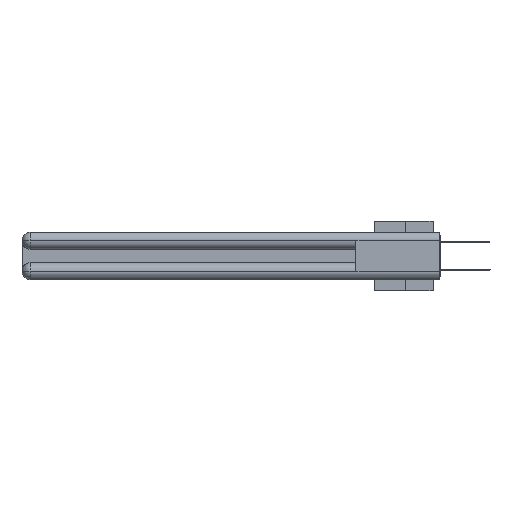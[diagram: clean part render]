
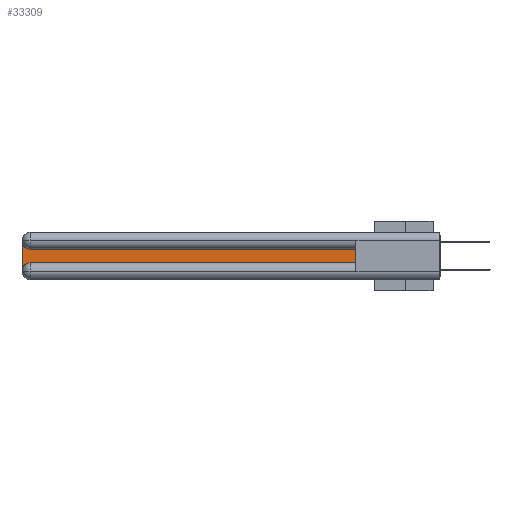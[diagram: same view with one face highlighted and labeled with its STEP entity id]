
A CAD part, left-side view. The second image highlights one B-rep face of the part: STEP entity #33309.
In plain terms, the highlighted planar face has unit normal (-1, 0, 0).
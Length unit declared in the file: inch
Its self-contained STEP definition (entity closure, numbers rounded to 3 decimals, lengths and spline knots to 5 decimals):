
#169 = DIRECTION ( 'NONE',  ( 0., 1., 0. ) ) ;
#691 = CARTESIAN_POINT ( 'NONE',  ( 0.075, 0.6, -0.2175 ) ) ;
#1352 = VECTOR ( 'NONE', #169, 39.37008 ) ;
#3128 = EDGE_CURVE ( 'NONE', #10000, #4557, #29777, .T. ) ;
#3247 = CARTESIAN_POINT ( 'NONE',  ( 0.075, 0.6, -0.2175 ) ) ;
#3289 = CARTESIAN_POINT ( 'NONE',  ( 0.075, 3., -0.1225 ) ) ;
#3720 = DIRECTION ( 'NONE',  ( 1., 0., 0. ) ) ;
#4289 = CARTESIAN_POINT ( 'NONE',  ( 0.075, 3., -0.2775 ) ) ;
#4380 = ORIENTED_EDGE ( 'NONE', *, *, #30515, .T. ) ;
#4533 = LINE ( 'NONE', #16848, #8865 ) ;
#4557 = VERTEX_POINT ( 'NONE', #12154 ) ;
#5357 = ORIENTED_EDGE ( 'NONE', *, *, #26463, .T. ) ;
#5626 = EDGE_CURVE ( 'NONE', #35240, #22213, #4533, .T. ) ;
#5837 = CIRCLE ( 'NONE', #23917, 0.06 ) ;
#6052 = VERTEX_POINT ( 'NONE', #20536 ) ;
#6240 = LINE ( 'NONE', #11932, #23591 ) ;
#6322 = DIRECTION ( 'NONE',  ( 0., 0., -1. ) ) ;
#6680 = VECTOR ( 'NONE', #30129, 39.37008 ) ;
#8865 = VECTOR ( 'NONE', #13929, 39.37008 ) ;
#9356 = ORIENTED_EDGE ( 'NONE', *, *, #15688, .T. ) ;
#10000 = VERTEX_POINT ( 'NONE', #25457 ) ;
#10992 = CARTESIAN_POINT ( 'NONE',  ( 0.075, 0.6, -0.1225 ) ) ;
#11683 = LINE ( 'NONE', #3247, #6680 ) ;
#11932 = CARTESIAN_POINT ( 'NONE',  ( 0.075, 3., -0.2175 ) ) ;
#12154 = CARTESIAN_POINT ( 'NONE',  ( 0.075, 2.94, -0.1225 ) ) ;
#13929 = DIRECTION ( 'NONE',  ( 0., -1., 0. ) ) ;
#14477 = AXIS2_PLACEMENT_3D ( 'NONE', #3289, #33278, #21062 ) ;
#15664 = ORIENTED_EDGE ( 'NONE', *, *, #3128, .T. ) ;
#15688 = EDGE_CURVE ( 'NONE', #6052, #34232, #6240, .T. ) ;
#16848 = CARTESIAN_POINT ( 'NONE',  ( 0.075, 0.6, -0.2175 ) ) ;
#18567 = EDGE_LOOP ( 'NONE', ( #15664, #28429, #9356, #4380, #30590, #5357 ) ) ;
#20536 = CARTESIAN_POINT ( 'NONE',  ( 0.075, 3., -0.0625 ) ) ;
#21062 = DIRECTION ( 'NONE',  ( 0., 0., -1. ) ) ;
#21448 = PLANE ( 'NONE',  #14477 ) ;
#21680 = CARTESIAN_POINT ( 'NONE',  ( 0.075, 2.94, -0.0625 ) ) ;
#22213 = VERTEX_POINT ( 'NONE', #691 ) ;
#23053 = AXIS2_PLACEMENT_3D ( 'NONE', #24832, #24655, #6322 ) ;
#23591 = VECTOR ( 'NONE', #23807, 39.37008 ) ;
#23807 = DIRECTION ( 'NONE',  ( 0., 0., -1. ) ) ;
#23823 = DIRECTION ( 'NONE',  ( 0., 0., -1. ) ) ;
#23917 = AXIS2_PLACEMENT_3D ( 'NONE', #21680, #3720, #23823 ) ;
#24146 = EDGE_CURVE ( 'NONE', #4557, #6052, #5837, .T. ) ;
#24655 = DIRECTION ( 'NONE',  ( 1., 0., 0. ) ) ;
#24832 = CARTESIAN_POINT ( 'NONE',  ( 0.075, 2.94, -0.2775 ) ) ;
#25457 = CARTESIAN_POINT ( 'NONE',  ( 0.075, 0.6, -0.1225 ) ) ;
#25613 = CARTESIAN_POINT ( 'NONE',  ( 0.075, 2.94, -0.2175 ) ) ;
#26463 = EDGE_CURVE ( 'NONE', #22213, #10000, #11683, .T. ) ;
#28429 = ORIENTED_EDGE ( 'NONE', *, *, #24146, .T. ) ;
#29777 = LINE ( 'NONE', #10992, #1352 ) ;
#29973 = FACE_OUTER_BOUND ( 'NONE', #18567, .T. ) ;
#30129 = DIRECTION ( 'NONE',  ( 0., 0., 1. ) ) ;
#30482 = CIRCLE ( 'NONE', #23053, 0.06 ) ;
#30515 = EDGE_CURVE ( 'NONE', #34232, #35240, #30482, .T. ) ;
#30590 = ORIENTED_EDGE ( 'NONE', *, *, #5626, .T. ) ;
#33278 = DIRECTION ( 'NONE',  ( 1., 0., 0. ) ) ;
#33309 = ADVANCED_FACE ( 'NONE', ( #29973 ), #21448, .F. ) ;
#34232 = VERTEX_POINT ( 'NONE', #4289 ) ;
#35240 = VERTEX_POINT ( 'NONE', #25613 ) ;
